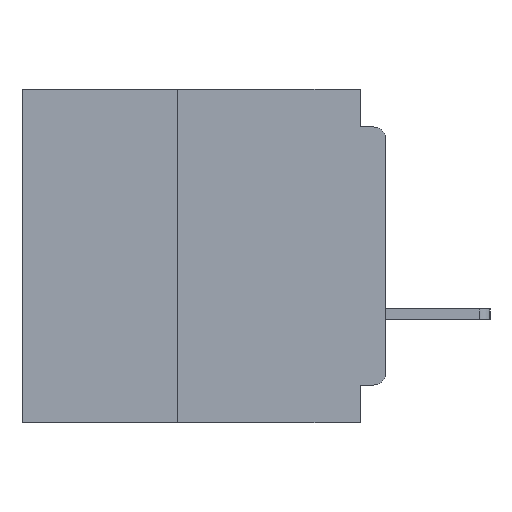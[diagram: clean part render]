
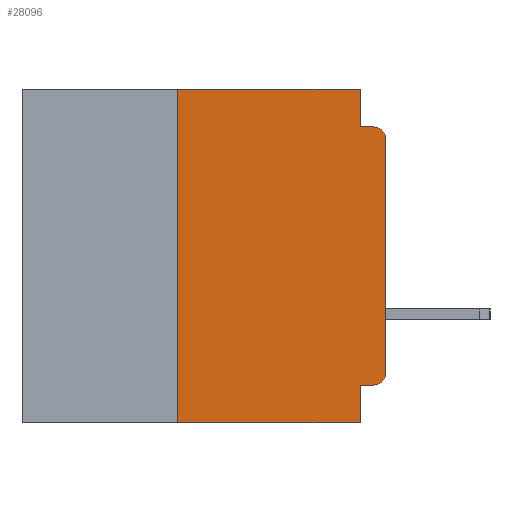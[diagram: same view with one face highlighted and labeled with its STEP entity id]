
A CAD part, left-side view. The second image highlights one B-rep face of the part: STEP entity #28096.
In plain terms, the highlighted planar face has unit normal (-1, 0, 0).
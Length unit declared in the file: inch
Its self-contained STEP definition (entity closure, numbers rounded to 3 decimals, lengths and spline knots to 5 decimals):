
#267 = CARTESIAN_POINT ( 'NONE',  ( 0., 0.015, -0.06 ) ) ;
#513 = DIRECTION ( 'NONE',  ( -1., 0., 0. ) ) ;
#566 = VECTOR ( 'NONE', #34909, 39.37008 ) ;
#613 = ORIENTED_EDGE ( 'NONE', *, *, #34593, .F. ) ;
#797 = VECTOR ( 'NONE', #5771, 39.37008 ) ;
#1110 = VECTOR ( 'NONE', #28228, 39.37008 ) ;
#1188 = CARTESIAN_POINT ( 'NONE',  ( 0., 0.437, 0. ) ) ;
#1295 = EDGE_CURVE ( 'NONE', #23249, #34496, #4723, .T. ) ;
#3092 = CARTESIAN_POINT ( 'NONE',  ( 0., 0.437, 0. ) ) ;
#3280 = DIRECTION ( 'NONE',  ( 0., 0., -1. ) ) ;
#3350 = CARTESIAN_POINT ( 'NONE',  ( 0., 0.25, -0.4 ) ) ;
#3352 = ORIENTED_EDGE ( 'NONE', *, *, #36559, .F. ) ;
#4679 = CARTESIAN_POINT ( 'NONE',  ( 0., 0., -0.045 ) ) ;
#4717 = CARTESIAN_POINT ( 'NONE',  ( 0., 0., -0.06 ) ) ;
#4723 = LINE ( 'NONE', #4679, #18922 ) ;
#4744 = CARTESIAN_POINT ( 'NONE',  ( 0., 0.031, -0.045 ) ) ;
#4939 = VECTOR ( 'NONE', #15115, 39.37008 ) ;
#5065 = EDGE_CURVE ( 'NONE', #27540, #36125, #17152, .T. ) ;
#5771 = DIRECTION ( 'NONE',  ( 0., -1., 0. ) ) ;
#5876 = ORIENTED_EDGE ( 'NONE', *, *, #1295, .F. ) ;
#6737 = CARTESIAN_POINT ( 'NONE',  ( 0., 0., 0. ) ) ;
#7878 = FACE_OUTER_BOUND ( 'NONE', #32882, .T. ) ;
#9485 = ORIENTED_EDGE ( 'NONE', *, *, #5065, .F. ) ;
#9575 = CARTESIAN_POINT ( 'NONE',  ( 0., 0.25, 0. ) ) ;
#10263 = EDGE_CURVE ( 'NONE', #21135, #30875, #20986, .T. ) ;
#10753 = DIRECTION ( 'NONE',  ( 0., -1., 0. ) ) ;
#11013 = EDGE_CURVE ( 'NONE', #15387, #38526, #38020, .T. ) ;
#12180 = DIRECTION ( 'NONE',  ( 1., 0., 0. ) ) ;
#14251 = AXIS2_PLACEMENT_3D ( 'NONE', #18592, #513, #21568 ) ;
#14405 = CIRCLE ( 'NONE', #33733, 0.015 ) ;
#15115 = DIRECTION ( 'NONE',  ( 0., 1., 0. ) ) ;
#15387 = VERTEX_POINT ( 'NONE', #33973 ) ;
#16105 = ORIENTED_EDGE ( 'NONE', *, *, #23525, .T. ) ;
#16938 = VECTOR ( 'NONE', #34085, 39.37008 ) ;
#16997 = ORIENTED_EDGE ( 'NONE', *, *, #29084, .T. ) ;
#17105 = EDGE_CURVE ( 'NONE', #21135, #15387, #26785, .T. ) ;
#17152 = LINE ( 'NONE', #1188, #1110 ) ;
#17555 = CARTESIAN_POINT ( 'NONE',  ( 0., 0.031, -0.355 ) ) ;
#18592 = CARTESIAN_POINT ( 'NONE',  ( 0., 0.015, -0.34 ) ) ;
#18660 = CARTESIAN_POINT ( 'NONE',  ( 0., 0.031, -0.4 ) ) ;
#18683 = CARTESIAN_POINT ( 'NONE',  ( 0., 0.031, 0. ) ) ;
#18922 = VECTOR ( 'NONE', #10753, 39.37008 ) ;
#18959 = CARTESIAN_POINT ( 'NONE',  ( 0., 0.031, -0.4 ) ) ;
#20986 = LINE ( 'NONE', #24053, #4939 ) ;
#21135 = VERTEX_POINT ( 'NONE', #24004 ) ;
#21329 = DIRECTION ( 'NONE',  ( -1., 0., 0. ) ) ;
#21568 = DIRECTION ( 'NONE',  ( 0., 0., -1. ) ) ;
#21800 = DIRECTION ( 'NONE',  ( 0., 0., -1. ) ) ;
#22392 = ORIENTED_EDGE ( 'NONE', *, *, #25700, .F. ) ;
#22719 = ORIENTED_EDGE ( 'NONE', *, *, #11013, .T. ) ;
#23249 = VERTEX_POINT ( 'NONE', #4744 ) ;
#23525 = EDGE_CURVE ( 'NONE', #38526, #34496, #14405, .T. ) ;
#23819 = CARTESIAN_POINT ( 'NONE',  ( 0., 0.437, -0.4 ) ) ;
#24004 = CARTESIAN_POINT ( 'NONE',  ( 0., 0.015, -0.355 ) ) ;
#24053 = CARTESIAN_POINT ( 'NONE',  ( 0., 0., -0.355 ) ) ;
#25700 = EDGE_CURVE ( 'NONE', #37680, #27540, #31787, .T. ) ;
#26189 = AXIS2_PLACEMENT_3D ( 'NONE', #3092, #12180, #33398 ) ;
#26785 = CIRCLE ( 'NONE', #14251, 0.015 ) ;
#27540 = VERTEX_POINT ( 'NONE', #9575 ) ;
#28096 = ADVANCED_FACE ( 'NONE', ( #7878 ), #36316, .F. ) ;
#28228 = DIRECTION ( 'NONE',  ( 0., -1., 0. ) ) ;
#28744 = CARTESIAN_POINT ( 'NONE',  ( 0., 0.25, -0.4 ) ) ;
#29084 = EDGE_CURVE ( 'NONE', #37680, #35218, #32015, .T. ) ;
#29683 = VECTOR ( 'NONE', #21800, 39.37008 ) ;
#29961 = VECTOR ( 'NONE', #37051, 39.37008 ) ;
#30875 = VERTEX_POINT ( 'NONE', #17555 ) ;
#31787 = LINE ( 'NONE', #28744, #566 ) ;
#32015 = LINE ( 'NONE', #23819, #797 ) ;
#32882 = EDGE_LOOP ( 'NONE', ( #22719, #16105, #5876, #613, #9485, #22392, #16997, #3352, #37898, #36325 ) ) ;
#33082 = LINE ( 'NONE', #18959, #16938 ) ;
#33398 = DIRECTION ( 'NONE',  ( 0., 0., -1. ) ) ;
#33733 = AXIS2_PLACEMENT_3D ( 'NONE', #267, #21329, #3280 ) ;
#33973 = CARTESIAN_POINT ( 'NONE',  ( 0., 0., -0.34 ) ) ;
#34085 = DIRECTION ( 'NONE',  ( 0., 0., -1. ) ) ;
#34496 = VERTEX_POINT ( 'NONE', #38258 ) ;
#34593 = EDGE_CURVE ( 'NONE', #36125, #23249, #38681, .T. ) ;
#34909 = DIRECTION ( 'NONE',  ( 0., 0., 1. ) ) ;
#35218 = VERTEX_POINT ( 'NONE', #18660 ) ;
#35307 = CARTESIAN_POINT ( 'NONE',  ( 0., 0.031, 0. ) ) ;
#36125 = VERTEX_POINT ( 'NONE', #35307 ) ;
#36316 = PLANE ( 'NONE',  #26189 ) ;
#36325 = ORIENTED_EDGE ( 'NONE', *, *, #17105, .T. ) ;
#36559 = EDGE_CURVE ( 'NONE', #30875, #35218, #33082, .T. ) ;
#37051 = DIRECTION ( 'NONE',  ( 0., 0., 1. ) ) ;
#37680 = VERTEX_POINT ( 'NONE', #3350 ) ;
#37898 = ORIENTED_EDGE ( 'NONE', *, *, #10263, .F. ) ;
#38020 = LINE ( 'NONE', #6737, #29961 ) ;
#38258 = CARTESIAN_POINT ( 'NONE',  ( 0., 0.015, -0.045 ) ) ;
#38526 = VERTEX_POINT ( 'NONE', #4717 ) ;
#38681 = LINE ( 'NONE', #18683, #29683 ) ;
